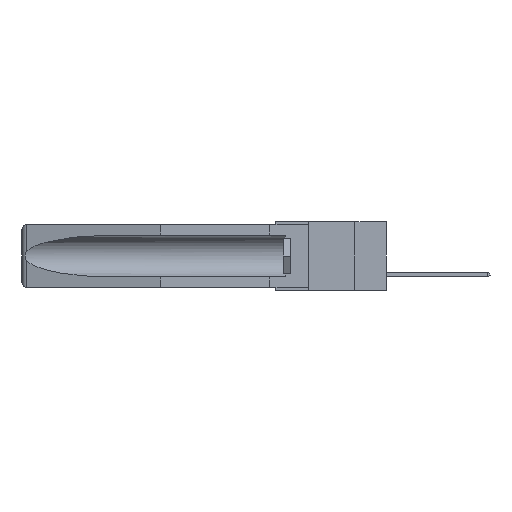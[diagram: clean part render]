
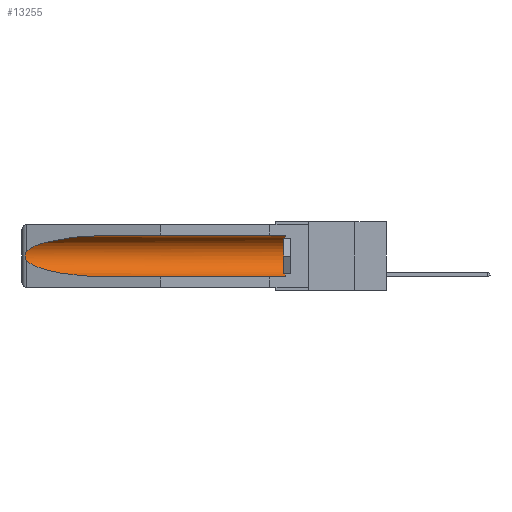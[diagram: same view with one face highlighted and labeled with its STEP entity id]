
A CAD part, left-side view. The second image highlights one B-rep face of the part: STEP entity #13255.
In plain terms, the highlighted cylindrical face has radius 2.857 mm (diameter 5.715 mm), a partial arc.
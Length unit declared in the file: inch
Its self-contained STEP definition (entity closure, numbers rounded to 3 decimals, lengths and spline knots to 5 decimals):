
#2 = VERTEX_POINT ( 'NONE', #8738 ) ;
#113 = DIRECTION ( 'NONE',  ( 0., 1., 0. ) ) ;
#253 = EDGE_LOOP ( 'NONE', ( #28212, #15397, #9740, #5839, #24445, #14252 ) ) ;
#340 = CARTESIAN_POINT ( 'NONE',  ( 0.2675, 1.53308, -0.16763 ) ) ;
#834 = VERTEX_POINT ( 'NONE', #22587 ) ;
#999 = CARTESIAN_POINT ( 'NONE',  ( 0.26655, 1.53094, -0.18657 ) ) ;
#1120 = CARTESIAN_POINT ( 'NONE',  ( 0.21114, 1.30732, -0.284 ) ) ;
#1547 = EDGE_CURVE ( 'NONE', #834, #26588, #7266, .T. ) ;
#2560 = VECTOR ( 'NONE', #12719, 39.37008 ) ;
#2665 = VECTOR ( 'NONE', #22959, 39.37008 ) ;
#4694 = CARTESIAN_POINT ( 'NONE',  ( 0.2673, 1.53269, -0.17917 ) ) ;
#5514 = CARTESIAN_POINT ( 'NONE',  ( 0.155, 0.126, -0.1715 ) ) ;
#5839 = ORIENTED_EDGE ( 'NONE', *, *, #17496, .F. ) ;
#6786 = EDGE_CURVE ( 'NONE', #24213, #834, #22733, .T. ) ;
#7052 = CARTESIAN_POINT ( 'NONE',  ( 0.26537, 1.52718, -0.14972 ) ) ;
#7266 =( BOUNDED_CURVE ( )  B_SPLINE_CURVE ( 3, ( #14258, #22902, #1120, #16426 ),
 .UNSPECIFIED., .F., .F. ) 
 B_SPLINE_CURVE_WITH_KNOTS ( ( 4, 4 ),
 ( 0.1948, 1.5708 ),
 .UNSPECIFIED. ) 
 CURVE ( )  GEOMETRIC_REPRESENTATION_ITEM ( )  RATIONAL_B_SPLINE_CURVE ( ( 1., 0.848, 0.848, 1. ) ) 
 REPRESENTATION_ITEM ( '' )  );
#8238 = EDGE_CURVE ( 'NONE', #2, #23413, #15147, .T. ) ;
#8738 = CARTESIAN_POINT ( 'NONE',  ( 0.155, 0.126, -0.284 ) ) ;
#9006 = CARTESIAN_POINT ( 'NONE',  ( 0.26597, 1.52961, -0.15275 ) ) ;
#9236 = CARTESIAN_POINT ( 'NONE',  ( 0.155, -0.30754, -0.1715 ) ) ;
#9740 = ORIENTED_EDGE ( 'NONE', *, *, #1547, .T. ) ;
#10083 = CARTESIAN_POINT ( 'NONE',  ( 0.21114, 1.30732, -0.059 ) ) ;
#11132 = AXIS2_PLACEMENT_3D ( 'NONE', #9236, #113, #13225 ) ;
#12158 = DIRECTION ( 'NONE',  ( 0., -1., 0. ) ) ;
#12719 = DIRECTION ( 'NONE',  ( 0., 1., 0. ) ) ;
#13225 = DIRECTION ( 'NONE',  ( 0., 0., 1. ) ) ;
#13255 = ADVANCED_FACE ( 'NONE', ( #18069 ), #23848, .F. ) ;
#13355 = CARTESIAN_POINT ( 'NONE',  ( 0.155, 0.126, -0.059 ) ) ;
#13465 = CARTESIAN_POINT ( 'NONE',  ( 0.2673, 1.5327, -0.16383 ) ) ;
#14252 = ORIENTED_EDGE ( 'NONE', *, *, #15944, .T. ) ;
#14258 = CARTESIAN_POINT ( 'NONE',  ( 0.26537, 1.52718, -0.19328 ) ) ;
#14282 = EDGE_CURVE ( 'NONE', #25744, #24213, #17671, .T. ) ;
#15147 = CIRCLE ( 'NONE', #24203, 0.1125 ) ;
#15299 = CARTESIAN_POINT ( 'NONE',  ( 0.155, -0.30754, -0.284 ) ) ;
#15397 = ORIENTED_EDGE ( 'NONE', *, *, #6786, .T. ) ;
#15637 = CARTESIAN_POINT ( 'NONE',  ( 0.2675, 1.53308, -0.17534 ) ) ;
#15930 = LINE ( 'NONE', #15299, #2560 ) ;
#15944 = EDGE_CURVE ( 'NONE', #23413, #25744, #23200, .T. ) ;
#16317 = CARTESIAN_POINT ( 'NONE',  ( 0.155, 1.07973, -0.059 ) ) ;
#16426 = CARTESIAN_POINT ( 'NONE',  ( 0.155, 1.07973, -0.284 ) ) ;
#17496 = EDGE_CURVE ( 'NONE', #2, #26588, #15930, .T. ) ;
#17671 =( BOUNDED_CURVE ( )  B_SPLINE_CURVE ( 3, ( #27766, #10083, #25384, #27658 ),
 .UNSPECIFIED., .F., .F. ) 
 B_SPLINE_CURVE_WITH_KNOTS ( ( 4, 4 ),
 ( 4.71239, 6.08839 ),
 .UNSPECIFIED. ) 
 CURVE ( )  GEOMETRIC_REPRESENTATION_ITEM ( )  RATIONAL_B_SPLINE_CURVE ( ( 1., 0.848, 0.848, 1. ) ) 
 REPRESENTATION_ITEM ( '' )  );
#18069 = FACE_OUTER_BOUND ( 'NONE', #253, .T. ) ;
#18681 = CARTESIAN_POINT ( 'NONE',  ( 0.155, -0.30754, -0.059 ) ) ;
#22587 = CARTESIAN_POINT ( 'NONE',  ( 0.26537, 1.52718, -0.19328 ) ) ;
#22733 = B_SPLINE_CURVE_WITH_KNOTS ( 'NONE', 3,
 ( #7052, #9006, #26511, #13465, #340, #15637, #4694, #999, #27264, #24795 ),
 .UNSPECIFIED., .F., .F.,
 ( 4, 2, 2, 2, 4 ),
 ( 0., 0.00029, 0.00058, 0.00087, 0.00117 ),
 .UNSPECIFIED. ) ;
#22902 = CARTESIAN_POINT ( 'NONE',  ( 0.25451, 1.48313, -0.24835 ) ) ;
#22959 = DIRECTION ( 'NONE',  ( 0., 1., 0. ) ) ;
#23200 = LINE ( 'NONE', #18681, #2665 ) ;
#23413 = VERTEX_POINT ( 'NONE', #13355 ) ;
#23848 = CYLINDRICAL_SURFACE ( 'NONE', #11132, 0.1125 ) ;
#24203 = AXIS2_PLACEMENT_3D ( 'NONE', #5514, #12158, #27222 ) ;
#24213 = VERTEX_POINT ( 'NONE', #25034 ) ;
#24445 = ORIENTED_EDGE ( 'NONE', *, *, #8238, .T. ) ;
#24795 = CARTESIAN_POINT ( 'NONE',  ( 0.26537, 1.52718, -0.19328 ) ) ;
#25034 = CARTESIAN_POINT ( 'NONE',  ( 0.26537, 1.52718, -0.14972 ) ) ;
#25384 = CARTESIAN_POINT ( 'NONE',  ( 0.25451, 1.48313, -0.09465 ) ) ;
#25744 = VERTEX_POINT ( 'NONE', #16317 ) ;
#26511 = CARTESIAN_POINT ( 'NONE',  ( 0.26654, 1.53092, -0.15636 ) ) ;
#26588 = VERTEX_POINT ( 'NONE', #28004 ) ;
#27222 = DIRECTION ( 'NONE',  ( 0., 0., 1. ) ) ;
#27264 = CARTESIAN_POINT ( 'NONE',  ( 0.26597, 1.5296, -0.19026 ) ) ;
#27658 = CARTESIAN_POINT ( 'NONE',  ( 0.26537, 1.52718, -0.14972 ) ) ;
#27766 = CARTESIAN_POINT ( 'NONE',  ( 0.155, 1.07973, -0.059 ) ) ;
#28004 = CARTESIAN_POINT ( 'NONE',  ( 0.155, 1.07973, -0.284 ) ) ;
#28212 = ORIENTED_EDGE ( 'NONE', *, *, #14282, .T. ) ;
